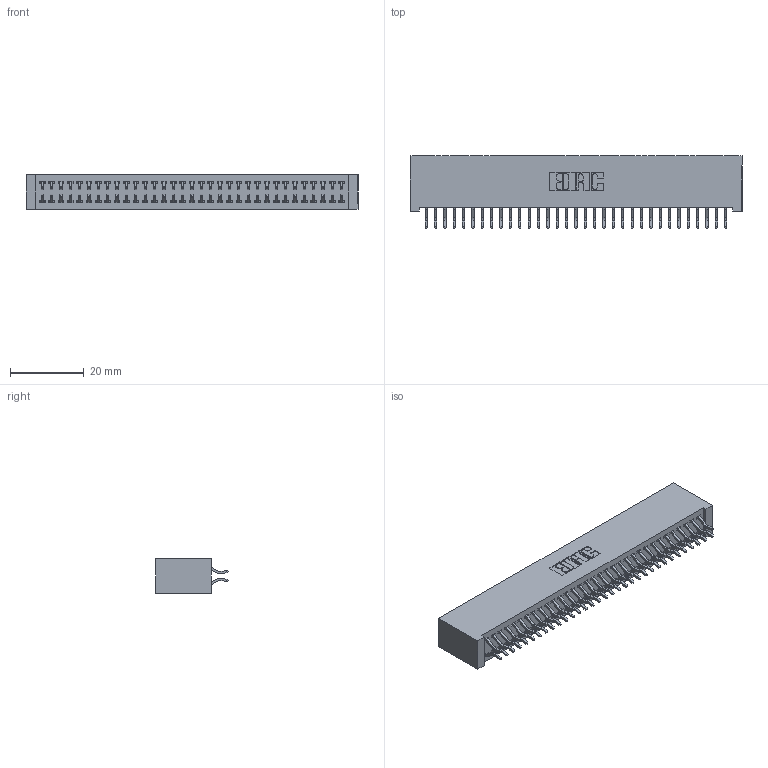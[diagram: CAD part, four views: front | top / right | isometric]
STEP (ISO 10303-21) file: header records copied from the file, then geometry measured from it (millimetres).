
FILE_DESCRIPTION (( 'STEP AP203' ), '1' );
FILE_NAME ('392-066-556-201.STEP', '2018-08-17T22:25:25', ( '' ), ( '' ), 'SwSTEP 2.0', 'SolidWorks 2016', '' );
FILE_SCHEMA (( 'CONFIG_CONTROL_DESIGN' ));
Length unit declared in the file: inch
Products named in the file (3): 342 Part_Lugless; 345-292-001_556 Tail; 392-066-556-201
Assembly tree (67 placements, depth 2):
  392-066-556-201
    342 Part_Lugless
    345-292-001_556 Tail  x66
Bounding box: 90.07 x 19.58 x 9.4 mm (x, y, z)
Volume: 8487.9 mm3; surface area: 13976.6 mm2
Topology: 67 solids, 67 shells, 3930 faces, 11693 edges, 7706 vertices
Faces by surface type: plane 2702, cylinder 1228
Entity records: 22205 total; most frequent: CARTESIAN_POINT 3702, ORIENTED_EDGE 3626, DIRECTION 3161, EDGE_CURVE 1813, LINE 1685, VECTOR 1685, VERTEX_POINT 1206, AXIS2_PLACEMENT_3D 738
